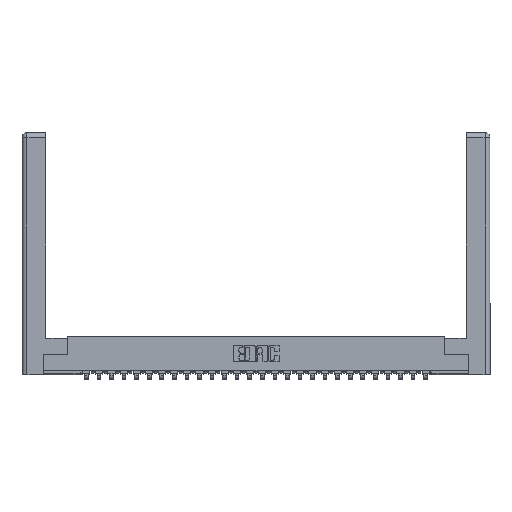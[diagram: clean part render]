
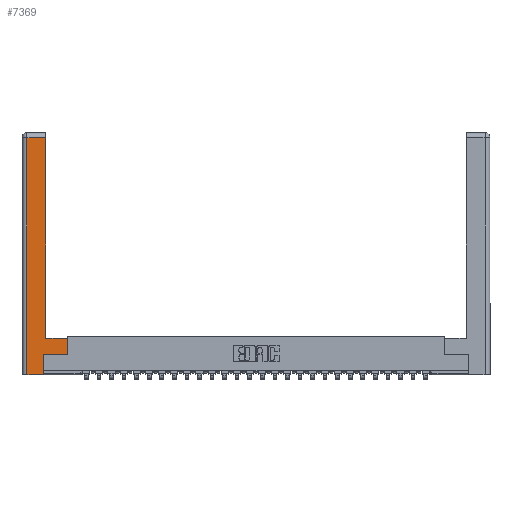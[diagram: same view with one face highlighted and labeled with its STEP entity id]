
A CAD part, top view. The second image highlights one B-rep face of the part: STEP entity #7369.
In plain terms, the highlighted planar face has unit normal (0, 0, 1).
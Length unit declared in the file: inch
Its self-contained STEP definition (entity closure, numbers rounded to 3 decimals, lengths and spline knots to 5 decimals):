
#363 = ORIENTED_EDGE ( 'NONE', *, *, #25909, .T. ) ;
#499 = VERTEX_POINT ( 'NONE', #2917 ) ;
#634 = ORIENTED_EDGE ( 'NONE', *, *, #15300, .T. ) ;
#1548 = CARTESIAN_POINT ( 'NONE',  ( 0.565, 0.45, 0. ) ) ;
#1863 = ORIENTED_EDGE ( 'NONE', *, *, #24325, .T. ) ;
#2158 = ORIENTED_EDGE ( 'NONE', *, *, #3051, .T. ) ;
#2917 = CARTESIAN_POINT ( 'NONE',  ( 0.265, 0.245, 0. ) ) ;
#3051 = EDGE_CURVE ( 'NONE', #18685, #7218, #17796, .T. ) ;
#3095 = FACE_OUTER_BOUND ( 'NONE', #20421, .T. ) ;
#3645 = VERTEX_POINT ( 'NONE', #7352 ) ;
#4056 = DIRECTION ( 'NONE',  ( 0., 1., 0. ) ) ;
#4876 = CARTESIAN_POINT ( 'NONE',  ( 0.0615, 0., 0. ) ) ;
#5048 = VERTEX_POINT ( 'NONE', #25164 ) ;
#5162 = CARTESIAN_POINT ( 'NONE',  ( 0., 0., 0. ) ) ;
#5336 = AXIS2_PLACEMENT_3D ( 'NONE', #5162, #14229, #23236 ) ;
#5778 = VECTOR ( 'NONE', #28737, 39.37008 ) ;
#5966 = DIRECTION ( 'NONE',  ( 0., 1., 0. ) ) ;
#6775 = DIRECTION ( 'NONE',  ( 0., 1., 0. ) ) ;
#7218 = VERTEX_POINT ( 'NONE', #4876 ) ;
#7352 = CARTESIAN_POINT ( 'NONE',  ( 0.565, 0.45, 0. ) ) ;
#7369 = ADVANCED_FACE ( 'NONE', ( #3095 ), #25447, .F. ) ;
#8493 = DIRECTION ( 'NONE',  ( -1., 0., 0. ) ) ;
#8647 = CARTESIAN_POINT ( 'NONE',  ( 0.0615, 2.94, 0. ) ) ;
#9361 = EDGE_CURVE ( 'NONE', #5048, #3645, #14892, .T. ) ;
#9837 = VECTOR ( 'NONE', #5966, 39.37008 ) ;
#10644 = CARTESIAN_POINT ( 'NONE',  ( 0.295, 0.45, 0. ) ) ;
#11061 = LINE ( 'NONE', #20088, #19371 ) ;
#11631 = DIRECTION ( 'NONE',  ( 1., 0., 0. ) ) ;
#12998 = LINE ( 'NONE', #13150, #28278 ) ;
#13019 = ORIENTED_EDGE ( 'NONE', *, *, #28889, .T. ) ;
#13150 = CARTESIAN_POINT ( 'NONE',  ( 0.265, 0.245, 0. ) ) ;
#13706 = VECTOR ( 'NONE', #4056, 39.37008 ) ;
#13909 = ORIENTED_EDGE ( 'NONE', *, *, #9361, .T. ) ;
#14229 = DIRECTION ( 'NONE',  ( 0., 0., -1. ) ) ;
#14776 = LINE ( 'NONE', #16843, #23183 ) ;
#14877 = VERTEX_POINT ( 'NONE', #20600 ) ;
#14892 = LINE ( 'NONE', #1548, #9837 ) ;
#15300 = EDGE_CURVE ( 'NONE', #499, #5048, #15572, .T. ) ;
#15428 = CARTESIAN_POINT ( 'NONE',  ( 0.265, 0., 0. ) ) ;
#15572 = LINE ( 'NONE', #24727, #23677 ) ;
#16263 = ORIENTED_EDGE ( 'NONE', *, *, #20036, .T. ) ;
#16843 = CARTESIAN_POINT ( 'NONE',  ( 0.295, 0.45, 0. ) ) ;
#17796 = LINE ( 'NONE', #28589, #5778 ) ;
#18685 = VERTEX_POINT ( 'NONE', #19367 ) ;
#19102 = EDGE_CURVE ( 'NONE', #25140, #499, #12998, .T. ) ;
#19367 = CARTESIAN_POINT ( 'NONE',  ( 0.0615, 2.94, 0. ) ) ;
#19371 = VECTOR ( 'NONE', #11631, 39.37008 ) ;
#19373 = VECTOR ( 'NONE', #8493, 39.37008 ) ;
#19491 = DIRECTION ( 'NONE',  ( -1., 0., 0. ) ) ;
#19620 = LINE ( 'NONE', #23651, #13706 ) ;
#20036 = EDGE_CURVE ( 'NONE', #14877, #18685, #24309, .T. ) ;
#20088 = CARTESIAN_POINT ( 'NONE',  ( 0.265, 0., 0. ) ) ;
#20421 = EDGE_LOOP ( 'NONE', ( #363, #16263, #2158, #1863, #21922, #634, #13909, #13019 ) ) ;
#20600 = CARTESIAN_POINT ( 'NONE',  ( 0.295, 2.94, 0. ) ) ;
#21922 = ORIENTED_EDGE ( 'NONE', *, *, #19102, .T. ) ;
#22101 = VERTEX_POINT ( 'NONE', #10644 ) ;
#23183 = VECTOR ( 'NONE', #19491, 39.37008 ) ;
#23236 = DIRECTION ( 'NONE',  ( -1., 0., 0. ) ) ;
#23651 = CARTESIAN_POINT ( 'NONE',  ( 0.295, 3., 0. ) ) ;
#23677 = VECTOR ( 'NONE', #27237, 39.37008 ) ;
#24309 = LINE ( 'NONE', #8647, #19373 ) ;
#24325 = EDGE_CURVE ( 'NONE', #7218, #25140, #11061, .T. ) ;
#24727 = CARTESIAN_POINT ( 'NONE',  ( 0.565, 0.245, 0. ) ) ;
#25140 = VERTEX_POINT ( 'NONE', #15428 ) ;
#25164 = CARTESIAN_POINT ( 'NONE',  ( 0.565, 0.245, 0. ) ) ;
#25447 = PLANE ( 'NONE',  #5336 ) ;
#25909 = EDGE_CURVE ( 'NONE', #22101, #14877, #19620, .T. ) ;
#27237 = DIRECTION ( 'NONE',  ( 1., 0., 0. ) ) ;
#28278 = VECTOR ( 'NONE', #6775, 39.37008 ) ;
#28589 = CARTESIAN_POINT ( 'NONE',  ( 0.0615, 0., 0. ) ) ;
#28737 = DIRECTION ( 'NONE',  ( 0., -1., 0. ) ) ;
#28889 = EDGE_CURVE ( 'NONE', #3645, #22101, #14776, .T. ) ;
